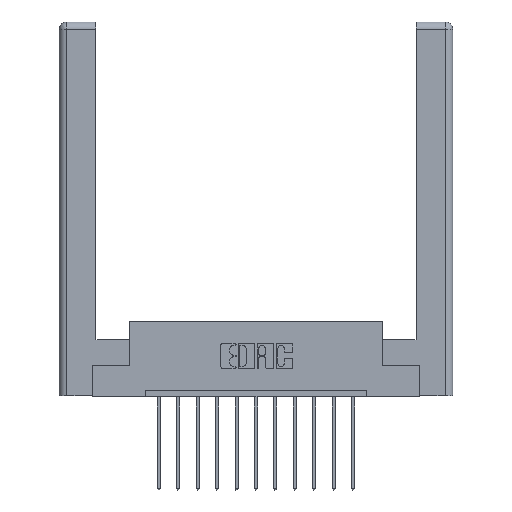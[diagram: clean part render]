
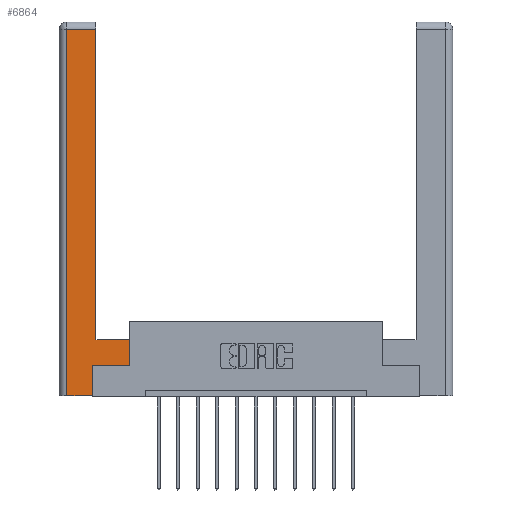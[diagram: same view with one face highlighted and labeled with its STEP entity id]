
A CAD part, top view. The second image highlights one B-rep face of the part: STEP entity #6864.
In plain terms, the highlighted planar face has unit normal (0, 0, 1).
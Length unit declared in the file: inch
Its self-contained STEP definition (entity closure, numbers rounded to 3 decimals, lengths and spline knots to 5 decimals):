
#117 = ORIENTED_EDGE ( 'NONE', *, *, #4960, .T. ) ;
#436 = CARTESIAN_POINT ( 'NONE',  ( 0.295, 3., 0. ) ) ;
#457 = VECTOR ( 'NONE', #9245, 39.37008 ) ;
#628 = EDGE_CURVE ( 'NONE', #13813, #2463, #7786, .T. ) ;
#730 = CARTESIAN_POINT ( 'NONE',  ( 0.565, 0.45, 0. ) ) ;
#1078 = ORIENTED_EDGE ( 'NONE', *, *, #9949, .T. ) ;
#1218 = DIRECTION ( 'NONE',  ( 0., -1., 0. ) ) ;
#1289 = CARTESIAN_POINT ( 'NONE',  ( 0.565, 0.245, 0. ) ) ;
#1425 = LINE ( 'NONE', #13275, #10393 ) ;
#1550 = DIRECTION ( 'NONE',  ( -1., 0., 0. ) ) ;
#1593 = EDGE_LOOP ( 'NONE', ( #12176, #11784, #117, #9003, #7400, #7303, #1078, #6600 ) ) ;
#1721 = CARTESIAN_POINT ( 'NONE',  ( 0.565, 0.245, 0. ) ) ;
#1757 = CARTESIAN_POINT ( 'NONE',  ( 0.565, 0.45, 0. ) ) ;
#1818 = DIRECTION ( 'NONE',  ( 0., 0., -1. ) ) ;
#1848 = LINE ( 'NONE', #13800, #10609 ) ;
#2006 = CARTESIAN_POINT ( 'NONE',  ( 0.0615, 0., 0. ) ) ;
#2463 = VERTEX_POINT ( 'NONE', #9144 ) ;
#3017 = CARTESIAN_POINT ( 'NONE',  ( 0.295, 2.94, 0. ) ) ;
#3658 = AXIS2_PLACEMENT_3D ( 'NONE', #5370, #1818, #13286 ) ;
#4105 = DIRECTION ( 'NONE',  ( 1., 0., 0. ) ) ;
#4805 = FACE_OUTER_BOUND ( 'NONE', #1593, .T. ) ;
#4960 = EDGE_CURVE ( 'NONE', #10358, #13405, #11654, .T. ) ;
#5370 = CARTESIAN_POINT ( 'NONE',  ( 0., 0., 0. ) ) ;
#5736 = EDGE_CURVE ( 'NONE', #12915, #8927, #14710, .T. ) ;
#5785 = CARTESIAN_POINT ( 'NONE',  ( 0.0615, 0., 0. ) ) ;
#5850 = CARTESIAN_POINT ( 'NONE',  ( 0.265, 0.245, 0. ) ) ;
#6199 = VERTEX_POINT ( 'NONE', #1721 ) ;
#6399 = VECTOR ( 'NONE', #12154, 39.37008 ) ;
#6600 = ORIENTED_EDGE ( 'NONE', *, *, #6755, .T. ) ;
#6755 = EDGE_CURVE ( 'NONE', #13376, #12915, #13223, .T. ) ;
#6864 = ADVANCED_FACE ( 'NONE', ( #4805 ), #7534, .F. ) ;
#7112 = VECTOR ( 'NONE', #1550, 39.37008 ) ;
#7303 = ORIENTED_EDGE ( 'NONE', *, *, #14837, .T. ) ;
#7400 = ORIENTED_EDGE ( 'NONE', *, *, #628, .T. ) ;
#7534 = PLANE ( 'NONE',  #3658 ) ;
#7786 = LINE ( 'NONE', #5850, #457 ) ;
#8263 = CARTESIAN_POINT ( 'NONE',  ( 0.295, 0.45, 0. ) ) ;
#8315 = CARTESIAN_POINT ( 'NONE',  ( 0.265, 0., 0. ) ) ;
#8927 = VERTEX_POINT ( 'NONE', #3017 ) ;
#9003 = ORIENTED_EDGE ( 'NONE', *, *, #14557, .T. ) ;
#9144 = CARTESIAN_POINT ( 'NONE',  ( 0.265, 0.245, 0. ) ) ;
#9161 = VECTOR ( 'NONE', #1218, 39.37008 ) ;
#9245 = DIRECTION ( 'NONE',  ( 0., 1., 0. ) ) ;
#9949 = EDGE_CURVE ( 'NONE', #6199, #13376, #13398, .T. ) ;
#10358 = VERTEX_POINT ( 'NONE', #11333 ) ;
#10393 = VECTOR ( 'NONE', #4105, 39.37008 ) ;
#10609 = VECTOR ( 'NONE', #12833, 39.37008 ) ;
#10640 = DIRECTION ( 'NONE',  ( 0., 1., 0. ) ) ;
#11333 = CARTESIAN_POINT ( 'NONE',  ( 0.0615, 2.94, 0. ) ) ;
#11654 = LINE ( 'NONE', #5785, #9161 ) ;
#11784 = ORIENTED_EDGE ( 'NONE', *, *, #12336, .T. ) ;
#11977 = CARTESIAN_POINT ( 'NONE',  ( 0.295, 0.45, 0. ) ) ;
#11978 = VECTOR ( 'NONE', #10640, 39.37008 ) ;
#12154 = DIRECTION ( 'NONE',  ( 0., 1., 0. ) ) ;
#12176 = ORIENTED_EDGE ( 'NONE', *, *, #5736, .T. ) ;
#12336 = EDGE_CURVE ( 'NONE', #8927, #10358, #1848, .T. ) ;
#12552 = VECTOR ( 'NONE', #13924, 39.37008 ) ;
#12833 = DIRECTION ( 'NONE',  ( -1., 0., 0. ) ) ;
#12907 = LINE ( 'NONE', #1289, #12552 ) ;
#12915 = VERTEX_POINT ( 'NONE', #11977 ) ;
#13223 = LINE ( 'NONE', #8263, #7112 ) ;
#13275 = CARTESIAN_POINT ( 'NONE',  ( 0.265, 0., 0. ) ) ;
#13286 = DIRECTION ( 'NONE',  ( -1., 0., 0. ) ) ;
#13376 = VERTEX_POINT ( 'NONE', #730 ) ;
#13398 = LINE ( 'NONE', #1757, #6399 ) ;
#13405 = VERTEX_POINT ( 'NONE', #2006 ) ;
#13800 = CARTESIAN_POINT ( 'NONE',  ( 0.0615, 2.94, 0. ) ) ;
#13813 = VERTEX_POINT ( 'NONE', #8315 ) ;
#13924 = DIRECTION ( 'NONE',  ( 1., 0., 0. ) ) ;
#14557 = EDGE_CURVE ( 'NONE', #13405, #13813, #1425, .T. ) ;
#14710 = LINE ( 'NONE', #436, #11978 ) ;
#14837 = EDGE_CURVE ( 'NONE', #2463, #6199, #12907, .T. ) ;
